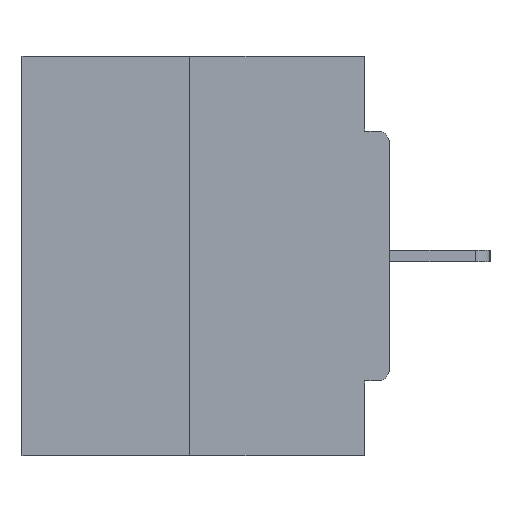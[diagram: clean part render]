
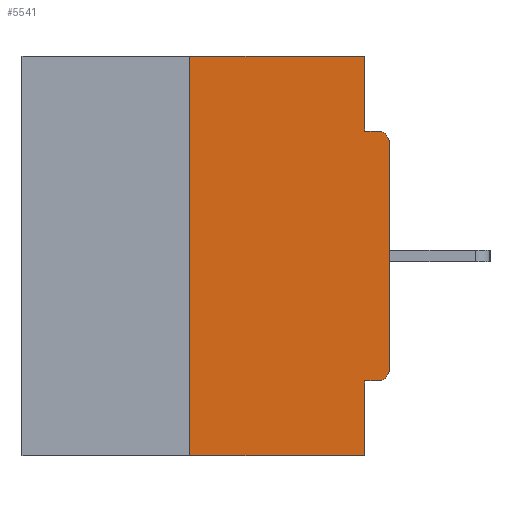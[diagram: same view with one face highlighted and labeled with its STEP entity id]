
A CAD part, left-side view. The second image highlights one B-rep face of the part: STEP entity #5541.
In plain terms, the highlighted planar face has unit normal (-1, 0, 0).
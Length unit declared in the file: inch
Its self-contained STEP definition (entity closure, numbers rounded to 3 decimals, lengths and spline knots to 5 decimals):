
#923 = LINE ( 'NONE', #9343, #13037 ) ;
#1434 = CARTESIAN_POINT ( 'NONE',  ( 0., 0.46, 0. ) ) ;
#2357 = DIRECTION ( 'NONE',  ( 0., 1., 0. ) ) ;
#3144 = DIRECTION ( 'NONE',  ( 0., 0., -1. ) ) ;
#3263 = CARTESIAN_POINT ( 'NONE',  ( 0., 0., -0.1085 ) ) ;
#3397 = AXIS2_PLACEMENT_3D ( 'NONE', #6701, #22149, #19662 ) ;
#3411 = ORIENTED_EDGE ( 'NONE', *, *, #25273, .F. ) ;
#3825 = EDGE_CURVE ( 'NONE', #21031, #20452, #20755, .T. ) ;
#3909 = CARTESIAN_POINT ( 'NONE',  ( 0., 0.015, -0.4065 ) ) ;
#4207 = VERTEX_POINT ( 'NONE', #8228 ) ;
#4441 = DIRECTION ( 'NONE',  ( 0., 0., 1. ) ) ;
#4570 = CARTESIAN_POINT ( 'NONE',  ( 0., 0., -0.0935 ) ) ;
#4859 = CARTESIAN_POINT ( 'NONE',  ( 0., 0., 0. ) ) ;
#5541 = ADVANCED_FACE ( 'NONE', ( #8279 ), #28731, .F. ) ;
#5831 = DIRECTION ( 'NONE',  ( 0., 0., -1. ) ) ;
#6701 = CARTESIAN_POINT ( 'NONE',  ( 0., 0.015, -0.1085 ) ) ;
#6793 = CARTESIAN_POINT ( 'NONE',  ( 0., 0.25, -0.5 ) ) ;
#6879 = ORIENTED_EDGE ( 'NONE', *, *, #26405, .T. ) ;
#7076 = CARTESIAN_POINT ( 'NONE',  ( 0., 0., -0.4065 ) ) ;
#7183 = LINE ( 'NONE', #14550, #23582 ) ;
#7657 = EDGE_CURVE ( 'NONE', #13232, #4207, #8357, .T. ) ;
#7685 = ORIENTED_EDGE ( 'NONE', *, *, #26364, .F. ) ;
#8174 = VECTOR ( 'NONE', #17343, 39.37008 ) ;
#8186 = VERTEX_POINT ( 'NONE', #13631 ) ;
#8228 = CARTESIAN_POINT ( 'NONE',  ( 0., 0.031, 0. ) ) ;
#8279 = FACE_OUTER_BOUND ( 'NONE', #18874, .T. ) ;
#8357 = LINE ( 'NONE', #1434, #8174 ) ;
#8566 = VECTOR ( 'NONE', #2357, 39.37008 ) ;
#8930 = ORIENTED_EDGE ( 'NONE', *, *, #25440, .T. ) ;
#9140 = LINE ( 'NONE', #4570, #28817 ) ;
#9343 = CARTESIAN_POINT ( 'NONE',  ( 0., 0.031, -0.5 ) ) ;
#9571 = DIRECTION ( 'NONE',  ( 0., -1., 0. ) ) ;
#10100 = LINE ( 'NONE', #14663, #20802 ) ;
#11581 = CARTESIAN_POINT ( 'NONE',  ( 0., 0.031, -0.5 ) ) ;
#11680 = CARTESIAN_POINT ( 'NONE',  ( 0., 0.25, 0. ) ) ;
#11737 = CARTESIAN_POINT ( 'NONE',  ( 0., 0., -0.3915 ) ) ;
#11865 = VERTEX_POINT ( 'NONE', #11581 ) ;
#12337 = CIRCLE ( 'NONE', #3397, 0.015 ) ;
#12570 = DIRECTION ( 'NONE',  ( 1., 0., 0. ) ) ;
#12600 = DIRECTION ( 'NONE',  ( 0., 0., -1. ) ) ;
#13037 = VECTOR ( 'NONE', #3144, 39.37008 ) ;
#13232 = VERTEX_POINT ( 'NONE', #18532 ) ;
#13446 = LINE ( 'NONE', #11680, #26259 ) ;
#13631 = CARTESIAN_POINT ( 'NONE',  ( 0., 0.015, -0.0935 ) ) ;
#13732 = VERTEX_POINT ( 'NONE', #19650 ) ;
#13738 = ORIENTED_EDGE ( 'NONE', *, *, #24350, .T. ) ;
#14063 = EDGE_CURVE ( 'NONE', #20452, #11865, #923, .T. ) ;
#14550 = CARTESIAN_POINT ( 'NONE',  ( 0., 0.031, 0. ) ) ;
#14663 = CARTESIAN_POINT ( 'NONE',  ( 0., 0.46, -0.5 ) ) ;
#14809 = DIRECTION ( 'NONE',  ( -1., 0., 0. ) ) ;
#15110 = CARTESIAN_POINT ( 'NONE',  ( 0., 0.031, -0.4065 ) ) ;
#17007 = DIRECTION ( 'NONE',  ( 0., -1., 0. ) ) ;
#17343 = DIRECTION ( 'NONE',  ( 0., -1., 0. ) ) ;
#17553 = DIRECTION ( 'NONE',  ( 0., 0., -1. ) ) ;
#17977 = EDGE_CURVE ( 'NONE', #24431, #13232, #13446, .T. ) ;
#18455 = ORIENTED_EDGE ( 'NONE', *, *, #7657, .F. ) ;
#18532 = CARTESIAN_POINT ( 'NONE',  ( 0., 0.25, 0. ) ) ;
#18874 = EDGE_LOOP ( 'NONE', ( #18455, #22238, #13738, #23504, #25778, #24365, #6879, #8930, #7685, #3411 ) ) ;
#19386 = AXIS2_PLACEMENT_3D ( 'NONE', #23341, #14809, #12600 ) ;
#19650 = CARTESIAN_POINT ( 'NONE',  ( 0., 0.031, -0.0935 ) ) ;
#19662 = DIRECTION ( 'NONE',  ( 0., 0., -1. ) ) ;
#20452 = VERTEX_POINT ( 'NONE', #15110 ) ;
#20752 = DIRECTION ( 'NONE',  ( 0., 0., 1. ) ) ;
#20755 = LINE ( 'NONE', #7076, #8566 ) ;
#20802 = VECTOR ( 'NONE', #17007, 39.37008 ) ;
#21031 = VERTEX_POINT ( 'NONE', #3909 ) ;
#22149 = DIRECTION ( 'NONE',  ( -1., 0., 0. ) ) ;
#22238 = ORIENTED_EDGE ( 'NONE', *, *, #17977, .F. ) ;
#23183 = AXIS2_PLACEMENT_3D ( 'NONE', #28296, #12570, #17553 ) ;
#23341 = CARTESIAN_POINT ( 'NONE',  ( 0., 0.015, -0.3915 ) ) ;
#23504 = ORIENTED_EDGE ( 'NONE', *, *, #14063, .F. ) ;
#23582 = VECTOR ( 'NONE', #5831, 39.37008 ) ;
#24235 = VERTEX_POINT ( 'NONE', #11737 ) ;
#24350 = EDGE_CURVE ( 'NONE', #24431, #11865, #10100, .T. ) ;
#24365 = ORIENTED_EDGE ( 'NONE', *, *, #24387, .T. ) ;
#24387 = EDGE_CURVE ( 'NONE', #21031, #24235, #26371, .T. ) ;
#24431 = VERTEX_POINT ( 'NONE', #6793 ) ;
#25020 = LINE ( 'NONE', #4859, #25073 ) ;
#25073 = VECTOR ( 'NONE', #20752, 39.37008 ) ;
#25273 = EDGE_CURVE ( 'NONE', #4207, #13732, #7183, .T. ) ;
#25440 = EDGE_CURVE ( 'NONE', #26166, #8186, #12337, .T. ) ;
#25778 = ORIENTED_EDGE ( 'NONE', *, *, #3825, .F. ) ;
#26166 = VERTEX_POINT ( 'NONE', #3263 ) ;
#26259 = VECTOR ( 'NONE', #4441, 39.37008 ) ;
#26364 = EDGE_CURVE ( 'NONE', #13732, #8186, #9140, .T. ) ;
#26371 = CIRCLE ( 'NONE', #19386, 0.015 ) ;
#26405 = EDGE_CURVE ( 'NONE', #24235, #26166, #25020, .T. ) ;
#28296 = CARTESIAN_POINT ( 'NONE',  ( 0., 0.46, 0. ) ) ;
#28731 = PLANE ( 'NONE',  #23183 ) ;
#28817 = VECTOR ( 'NONE', #9571, 39.37008 ) ;
